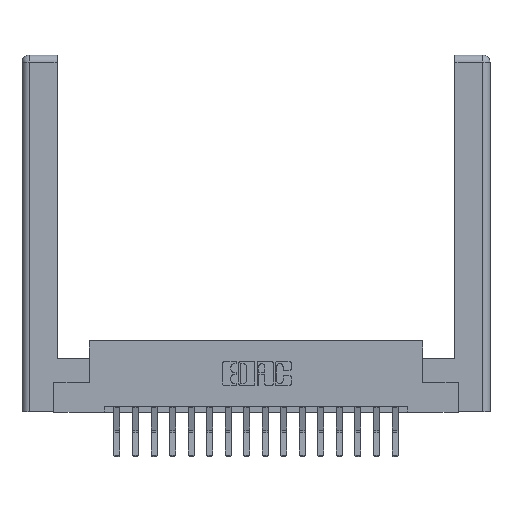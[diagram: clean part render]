
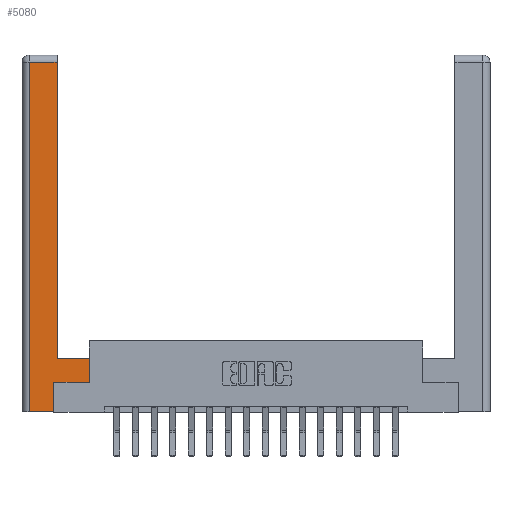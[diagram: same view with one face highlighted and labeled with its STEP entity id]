
A CAD part, top view. The second image highlights one B-rep face of the part: STEP entity #5080.
In plain terms, the highlighted planar face has unit normal (0, 0, 1).
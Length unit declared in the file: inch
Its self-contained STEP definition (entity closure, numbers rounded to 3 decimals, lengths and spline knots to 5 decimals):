
#30 = DIRECTION ( 'NONE',  ( 0., 1., 0. ) ) ;
#401 = DIRECTION ( 'NONE',  ( 0., 1., 0. ) ) ;
#439 = VERTEX_POINT ( 'NONE', #14872 ) ;
#494 = CARTESIAN_POINT ( 'NONE',  ( 0.265, 0., 0. ) ) ;
#547 = VERTEX_POINT ( 'NONE', #8133 ) ;
#1300 = ORIENTED_EDGE ( 'NONE', *, *, #17944, .T. ) ;
#1559 = VECTOR ( 'NONE', #2386, 39.37008 ) ;
#2013 = LINE ( 'NONE', #5119, #1559 ) ;
#2018 = DIRECTION ( 'NONE',  ( -1., 0., 0. ) ) ;
#2192 = EDGE_CURVE ( 'NONE', #547, #9110, #15137, .T. ) ;
#2386 = DIRECTION ( 'NONE',  ( 0., -1., 0. ) ) ;
#2644 = LINE ( 'NONE', #17380, #13553 ) ;
#2763 = EDGE_CURVE ( 'NONE', #16927, #9394, #15529, .T. ) ;
#2940 = ORIENTED_EDGE ( 'NONE', *, *, #2192, .T. ) ;
#3015 = DIRECTION ( 'NONE',  ( 0., 1., 0. ) ) ;
#3410 = CARTESIAN_POINT ( 'NONE',  ( 0.265, 0., 0. ) ) ;
#3623 = CARTESIAN_POINT ( 'NONE',  ( 0.565, 0.245, 0. ) ) ;
#4660 = LINE ( 'NONE', #3623, #15172 ) ;
#5080 = ADVANCED_FACE ( 'NONE', ( #7194 ), #13119, .F. ) ;
#5119 = CARTESIAN_POINT ( 'NONE',  ( 0.0615, 0., 0. ) ) ;
#6041 = DIRECTION ( 'NONE',  ( -1., 0., 0. ) ) ;
#6218 = DIRECTION ( 'NONE',  ( 1., 0., 0. ) ) ;
#6505 = ORIENTED_EDGE ( 'NONE', *, *, #17617, .T. ) ;
#6607 = VECTOR ( 'NONE', #2018, 39.37008 ) ;
#7060 = ORIENTED_EDGE ( 'NONE', *, *, #2763, .T. ) ;
#7194 = FACE_OUTER_BOUND ( 'NONE', #9808, .T. ) ;
#7384 = VECTOR ( 'NONE', #30, 39.37008 ) ;
#7764 = VERTEX_POINT ( 'NONE', #16650 ) ;
#7945 = ORIENTED_EDGE ( 'NONE', *, *, #8705, .T. ) ;
#8133 = CARTESIAN_POINT ( 'NONE',  ( 0.0615, 0., 0. ) ) ;
#8179 = EDGE_CURVE ( 'NONE', #9110, #7764, #8920, .T. ) ;
#8598 = CARTESIAN_POINT ( 'NONE',  ( 0.565, 0.45, 0. ) ) ;
#8705 = EDGE_CURVE ( 'NONE', #9394, #439, #14259, .T. ) ;
#8920 = LINE ( 'NONE', #17227, #12480 ) ;
#9110 = VERTEX_POINT ( 'NONE', #3410 ) ;
#9191 = DIRECTION ( 'NONE',  ( -1., 0., 0. ) ) ;
#9394 = VERTEX_POINT ( 'NONE', #16870 ) ;
#9462 = EDGE_CURVE ( 'NONE', #439, #16894, #2644, .T. ) ;
#9808 = EDGE_LOOP ( 'NONE', ( #7945, #14182, #14352, #2940, #11784, #1300, #6505, #7060 ) ) ;
#11320 = VECTOR ( 'NONE', #6218, 39.37008 ) ;
#11763 = DIRECTION ( 'NONE',  ( 0., 0., -1. ) ) ;
#11784 = ORIENTED_EDGE ( 'NONE', *, *, #8179, .T. ) ;
#12480 = VECTOR ( 'NONE', #3015, 39.37008 ) ;
#12802 = CARTESIAN_POINT ( 'NONE',  ( 0.565, 0.245, 0. ) ) ;
#13119 = PLANE ( 'NONE',  #15485 ) ;
#13221 = CARTESIAN_POINT ( 'NONE',  ( 0.295, 3., 0. ) ) ;
#13365 = LINE ( 'NONE', #8598, #7384 ) ;
#13553 = VECTOR ( 'NONE', #9191, 39.37008 ) ;
#13671 = CARTESIAN_POINT ( 'NONE',  ( 0.565, 0.45, 0. ) ) ;
#13789 = VERTEX_POINT ( 'NONE', #12802 ) ;
#14182 = ORIENTED_EDGE ( 'NONE', *, *, #9462, .T. ) ;
#14259 = LINE ( 'NONE', #13221, #15830 ) ;
#14352 = ORIENTED_EDGE ( 'NONE', *, *, #17966, .T. ) ;
#14587 = CARTESIAN_POINT ( 'NONE',  ( 0., 0., 0. ) ) ;
#14872 = CARTESIAN_POINT ( 'NONE',  ( 0.295, 2.94, 0. ) ) ;
#15137 = LINE ( 'NONE', #494, #11320 ) ;
#15172 = VECTOR ( 'NONE', #17889, 39.37008 ) ;
#15249 = CARTESIAN_POINT ( 'NONE',  ( 0.0615, 2.94, 0. ) ) ;
#15485 = AXIS2_PLACEMENT_3D ( 'NONE', #14587, #11763, #6041 ) ;
#15529 = LINE ( 'NONE', #17686, #6607 ) ;
#15830 = VECTOR ( 'NONE', #401, 39.37008 ) ;
#16650 = CARTESIAN_POINT ( 'NONE',  ( 0.265, 0.245, 0. ) ) ;
#16870 = CARTESIAN_POINT ( 'NONE',  ( 0.295, 0.45, 0. ) ) ;
#16894 = VERTEX_POINT ( 'NONE', #15249 ) ;
#16927 = VERTEX_POINT ( 'NONE', #13671 ) ;
#17227 = CARTESIAN_POINT ( 'NONE',  ( 0.265, 0.245, 0. ) ) ;
#17380 = CARTESIAN_POINT ( 'NONE',  ( 0.0615, 2.94, 0. ) ) ;
#17617 = EDGE_CURVE ( 'NONE', #13789, #16927, #13365, .T. ) ;
#17686 = CARTESIAN_POINT ( 'NONE',  ( 0.295, 0.45, 0. ) ) ;
#17889 = DIRECTION ( 'NONE',  ( 1., 0., 0. ) ) ;
#17944 = EDGE_CURVE ( 'NONE', #7764, #13789, #4660, .T. ) ;
#17966 = EDGE_CURVE ( 'NONE', #16894, #547, #2013, .T. ) ;
